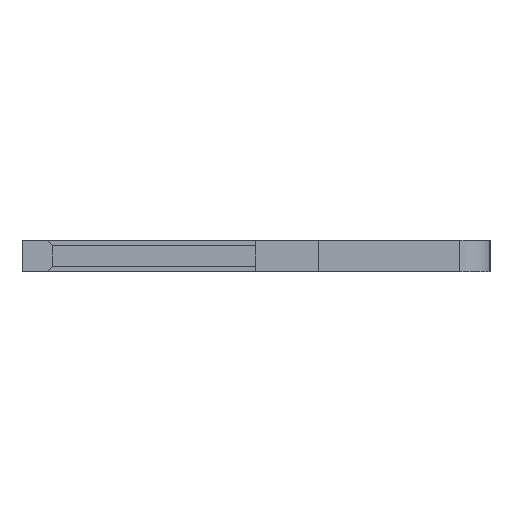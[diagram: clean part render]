
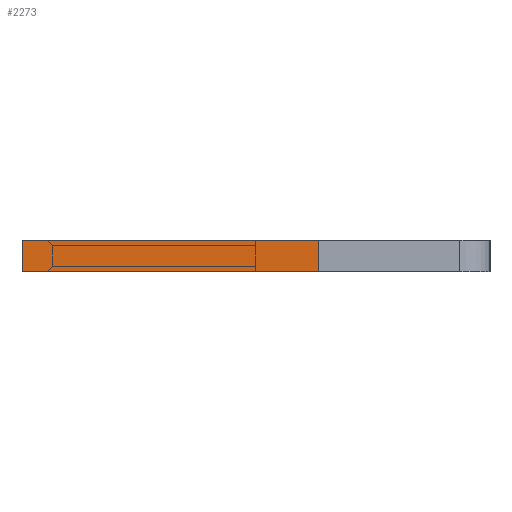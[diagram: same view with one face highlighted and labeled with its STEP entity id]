
A CAD part, left-side view. The second image highlights one B-rep face of the part: STEP entity #2273.
In plain terms, the highlighted face is planar.
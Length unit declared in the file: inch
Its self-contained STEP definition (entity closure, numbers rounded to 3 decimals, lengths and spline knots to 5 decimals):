
#93 = CARTESIAN_POINT ( 'NONE',  ( 0.01, 0.15, -0.04 ) ) ;
#123 = DIRECTION ( 'NONE',  ( 0., 1., 0. ) ) ;
#143 = EDGE_CURVE ( 'NONE', #1976, #317, #690, .T. ) ;
#317 = VERTEX_POINT ( 'NONE', #2708 ) ;
#329 = CARTESIAN_POINT ( 'NONE',  ( -0.01, -0.04, -0.04 ) ) ;
#368 = VERTEX_POINT ( 'NONE', #2389 ) ;
#454 = ORIENTED_EDGE ( 'NONE', *, *, #143, .T. ) ;
#690 = LINE ( 'NONE', #2641, #790 ) ;
#691 = DIRECTION ( 'NONE',  ( 0., 1., 0. ) ) ;
#790 = VECTOR ( 'NONE', #123, 39.37008 ) ;
#923 = LINE ( 'NONE', #93, #3044 ) ;
#976 = ORIENTED_EDGE ( 'NONE', *, *, #2258, .T. ) ;
#1302 = PLANE ( 'NONE',  #2102 ) ;
#1641 = CARTESIAN_POINT ( 'NONE',  ( 0.01, 0.15, -0.04 ) ) ;
#1780 = VECTOR ( 'NONE', #2533, 39.37008 ) ;
#1928 = DIRECTION ( 'NONE',  ( 1., 0., 0. ) ) ;
#1976 = VERTEX_POINT ( 'NONE', #329 ) ;
#2085 = VERTEX_POINT ( 'NONE', #2805 ) ;
#2102 = AXIS2_PLACEMENT_3D ( 'NONE', #3490, #2855, #1928 ) ;
#2121 = LINE ( 'NONE', #3158, #3572 ) ;
#2214 = LINE ( 'NONE', #1641, #1780 ) ;
#2258 = EDGE_CURVE ( 'NONE', #2085, #1976, #2121, .T. ) ;
#2273 = ADVANCED_FACE ( 'NONE', ( #2557 ), #1302, .F. ) ;
#2389 = CARTESIAN_POINT ( 'NONE',  ( 0.01, 0.15, -0.04 ) ) ;
#2496 = EDGE_CURVE ( 'NONE', #2085, #368, #923, .T. ) ;
#2533 = DIRECTION ( 'NONE',  ( -1., 0., 0. ) ) ;
#2557 = FACE_OUTER_BOUND ( 'NONE', #2571, .T. ) ;
#2571 = EDGE_LOOP ( 'NONE', ( #454, #2822, #3583, #976 ) ) ;
#2641 = CARTESIAN_POINT ( 'NONE',  ( -0.01, 0.15, -0.04 ) ) ;
#2708 = CARTESIAN_POINT ( 'NONE',  ( -0.01, 0.15, -0.04 ) ) ;
#2767 = EDGE_CURVE ( 'NONE', #368, #317, #2214, .T. ) ;
#2805 = CARTESIAN_POINT ( 'NONE',  ( 0.01, -0.04, -0.04 ) ) ;
#2822 = ORIENTED_EDGE ( 'NONE', *, *, #2767, .F. ) ;
#2855 = DIRECTION ( 'NONE',  ( 0., 0., 1. ) ) ;
#3044 = VECTOR ( 'NONE', #691, 39.37008 ) ;
#3158 = CARTESIAN_POINT ( 'NONE',  ( 0.01, -0.04, -0.04 ) ) ;
#3490 = CARTESIAN_POINT ( 'NONE',  ( 0.01, 0.15, -0.04 ) ) ;
#3572 = VECTOR ( 'NONE', #3776, 39.37008 ) ;
#3583 = ORIENTED_EDGE ( 'NONE', *, *, #2496, .F. ) ;
#3776 = DIRECTION ( 'NONE',  ( -1., 0., 0. ) ) ;
